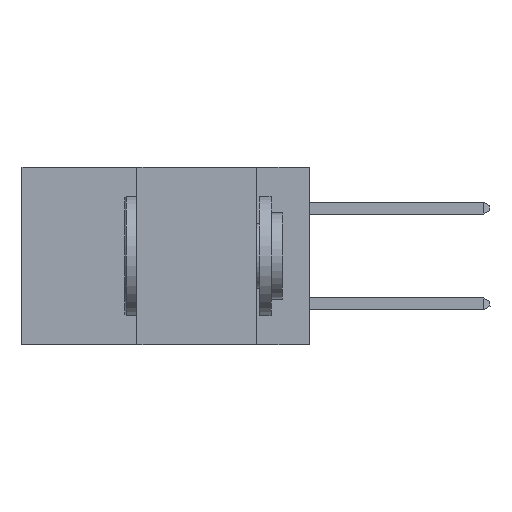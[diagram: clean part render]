
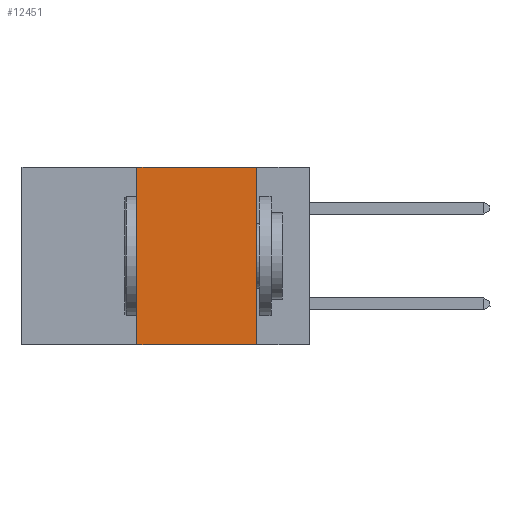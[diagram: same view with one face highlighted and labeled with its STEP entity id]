
A CAD part, left-side view. The second image highlights one B-rep face of the part: STEP entity #12451.
In plain terms, the highlighted planar face has unit normal (-1, 0, 0).
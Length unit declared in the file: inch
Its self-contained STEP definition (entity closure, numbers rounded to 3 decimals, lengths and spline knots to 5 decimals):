
#2340 = DIRECTION ( 'NONE',  ( 1., 0., 0. ) ) ;
#2652 = EDGE_CURVE ( 'NONE', #19748, #16121, #8352, .T. ) ;
#2740 = DIRECTION ( 'NONE',  ( 0., -1., 0. ) ) ;
#3579 = LINE ( 'NONE', #13608, #13181 ) ;
#4415 = EDGE_LOOP ( 'NONE', ( #20670, #8109, #9785, #16840 ) ) ;
#5493 = CARTESIAN_POINT ( 'NONE',  ( 0., 0.11, 0. ) ) ;
#5531 = AXIS2_PLACEMENT_3D ( 'NONE', #22011, #2340, #14997 ) ;
#5690 = DIRECTION ( 'NONE',  ( 0., -1., 0. ) ) ;
#8109 = ORIENTED_EDGE ( 'NONE', *, *, #13430, .F. ) ;
#8352 = LINE ( 'NONE', #21949, #22024 ) ;
#9785 = ORIENTED_EDGE ( 'NONE', *, *, #11603, .F. ) ;
#11011 = CARTESIAN_POINT ( 'NONE',  ( 0., 0.6, -0.37 ) ) ;
#11603 = EDGE_CURVE ( 'NONE', #18494, #22768, #14394, .T. ) ;
#11711 = EDGE_CURVE ( 'NONE', #18494, #16121, #21531, .T. ) ;
#12122 = VECTOR ( 'NONE', #5690, 39.37008 ) ;
#12225 = CARTESIAN_POINT ( 'NONE',  ( 0., 0.36, 0. ) ) ;
#12451 = ADVANCED_FACE ( 'NONE', ( #15445 ), #13219, .F. ) ;
#13181 = VECTOR ( 'NONE', #2740, 39.37008 ) ;
#13219 = PLANE ( 'NONE',  #5531 ) ;
#13430 = EDGE_CURVE ( 'NONE', #22768, #19748, #3579, .T. ) ;
#13608 = CARTESIAN_POINT ( 'NONE',  ( 0., 0.6, 0. ) ) ;
#14394 = LINE ( 'NONE', #12225, #19053 ) ;
#14997 = DIRECTION ( 'NONE',  ( 0., 0., -1. ) ) ;
#15445 = FACE_OUTER_BOUND ( 'NONE', #4415, .T. ) ;
#16121 = VERTEX_POINT ( 'NONE', #18847 ) ;
#16840 = ORIENTED_EDGE ( 'NONE', *, *, #11711, .T. ) ;
#17601 = CARTESIAN_POINT ( 'NONE',  ( 0., 0.36, -0.37 ) ) ;
#18494 = VERTEX_POINT ( 'NONE', #17601 ) ;
#18847 = CARTESIAN_POINT ( 'NONE',  ( 0., 0.11, -0.37 ) ) ;
#19053 = VECTOR ( 'NONE', #22820, 39.37008 ) ;
#19748 = VERTEX_POINT ( 'NONE', #5493 ) ;
#20670 = ORIENTED_EDGE ( 'NONE', *, *, #2652, .F. ) ;
#21531 = LINE ( 'NONE', #11011, #12122 ) ;
#21876 = DIRECTION ( 'NONE',  ( 0., 0., -1. ) ) ;
#21949 = CARTESIAN_POINT ( 'NONE',  ( 0., 0.11, 0. ) ) ;
#22011 = CARTESIAN_POINT ( 'NONE',  ( 0., 0.6, 0. ) ) ;
#22024 = VECTOR ( 'NONE', #21876, 39.37008 ) ;
#22454 = CARTESIAN_POINT ( 'NONE',  ( 0., 0.36, 0. ) ) ;
#22768 = VERTEX_POINT ( 'NONE', #22454 ) ;
#22820 = DIRECTION ( 'NONE',  ( 0., 0., 1. ) ) ;
